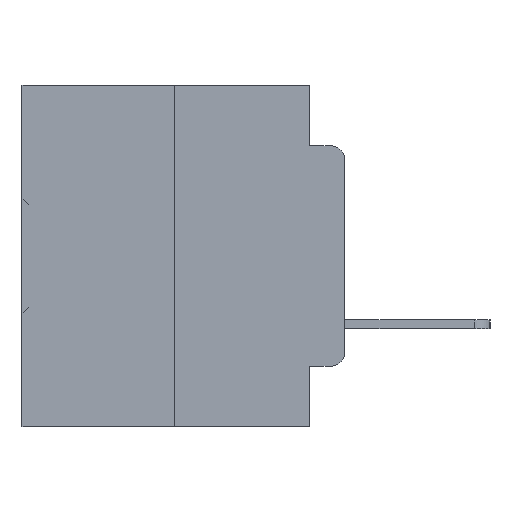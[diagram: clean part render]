
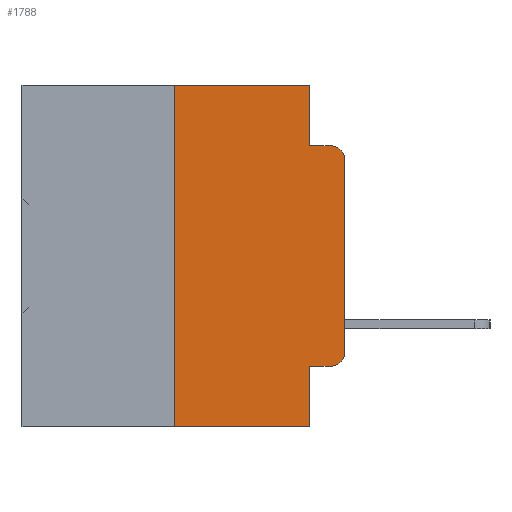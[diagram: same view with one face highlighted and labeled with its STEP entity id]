
A CAD part, left-side view. The second image highlights one B-rep face of the part: STEP entity #1788.
In plain terms, the highlighted planar face has unit normal (-1, 0, 0).
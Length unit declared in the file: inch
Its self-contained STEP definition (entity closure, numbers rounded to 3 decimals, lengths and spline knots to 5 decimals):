
#322 = CARTESIAN_POINT ( 'NONE',  ( 0., 0., -0.3915 ) ) ;
#651 = VECTOR ( 'NONE', #25806, 39.37008 ) ;
#716 = ORIENTED_EDGE ( 'NONE', *, *, #27039, .T. ) ;
#754 = DIRECTION ( 'NONE',  ( 0., -1., 0. ) ) ;
#1628 = CARTESIAN_POINT ( 'NONE',  ( 0., 0.25, 0. ) ) ;
#1788 = ADVANCED_FACE ( 'NONE', ( #13423 ), #5880, .F. ) ;
#2071 = VERTEX_POINT ( 'NONE', #32839 ) ;
#2243 = LINE ( 'NONE', #10859, #23206 ) ;
#2518 = CIRCLE ( 'NONE', #29534, 0.02 ) ;
#3226 = ORIENTED_EDGE ( 'NONE', *, *, #8585, .F. ) ;
#4117 = CARTESIAN_POINT ( 'NONE',  ( 0., 0.051, -0.0885 ) ) ;
#4327 = VERTEX_POINT ( 'NONE', #17687 ) ;
#4739 = DIRECTION ( 'NONE',  ( 0., 0., -1. ) ) ;
#5241 = DIRECTION ( 'NONE',  ( -1., 0., 0. ) ) ;
#5880 = PLANE ( 'NONE',  #23293 ) ;
#6751 = CARTESIAN_POINT ( 'NONE',  ( 0., 0.051, -0.4115 ) ) ;
#6845 = VERTEX_POINT ( 'NONE', #28659 ) ;
#7398 = LINE ( 'NONE', #20238, #21062 ) ;
#7960 = LINE ( 'NONE', #6751, #651 ) ;
#8549 = DIRECTION ( 'NONE',  ( 0., 0., -1. ) ) ;
#8585 = EDGE_CURVE ( 'NONE', #31777, #33695, #7398, .T. ) ;
#8704 = DIRECTION ( 'NONE',  ( 0., 0., -1. ) ) ;
#10718 = DIRECTION ( 'NONE',  ( 0., -1., 0. ) ) ;
#10859 = CARTESIAN_POINT ( 'NONE',  ( 0., 0., 0. ) ) ;
#11334 = DIRECTION ( 'NONE',  ( 1., 0., 0. ) ) ;
#11794 = DIRECTION ( 'NONE',  ( -1., 0., 0. ) ) ;
#12332 = EDGE_CURVE ( 'NONE', #2071, #6845, #7960, .T. ) ;
#12354 = LINE ( 'NONE', #27986, #25967 ) ;
#12371 = DIRECTION ( 'NONE',  ( 0., -1., 0. ) ) ;
#13351 = VERTEX_POINT ( 'NONE', #322 ) ;
#13352 = CARTESIAN_POINT ( 'NONE',  ( 0., 0.051, 0. ) ) ;
#13423 = FACE_OUTER_BOUND ( 'NONE', #16898, .T. ) ;
#13472 = EDGE_CURVE ( 'NONE', #6845, #13351, #27029, .T. ) ;
#13882 = VERTEX_POINT ( 'NONE', #32390 ) ;
#14518 = DIRECTION ( 'NONE',  ( 0., 0., 1. ) ) ;
#14878 = EDGE_CURVE ( 'NONE', #2071, #4327, #18936, .T. ) ;
#15846 = VERTEX_POINT ( 'NONE', #20016 ) ;
#16189 = EDGE_CURVE ( 'NONE', #15846, #13882, #2518, .T. ) ;
#16545 = ORIENTED_EDGE ( 'NONE', *, *, #29329, .F. ) ;
#16795 = CARTESIAN_POINT ( 'NONE',  ( 0., 0.473, 0. ) ) ;
#16898 = EDGE_LOOP ( 'NONE', ( #716, #28447, #17100, #18820, #3226, #16545, #24313, #28804, #24679, #28903 ) ) ;
#17100 = ORIENTED_EDGE ( 'NONE', *, *, #19858, .F. ) ;
#17377 = VECTOR ( 'NONE', #754, 39.37008 ) ;
#17687 = CARTESIAN_POINT ( 'NONE',  ( 0., 0.051, -0.5 ) ) ;
#17875 = EDGE_CURVE ( 'NONE', #33695, #21159, #27769, .T. ) ;
#18107 = VECTOR ( 'NONE', #4739, 39.37008 ) ;
#18820 = ORIENTED_EDGE ( 'NONE', *, *, #17875, .F. ) ;
#18852 = CARTESIAN_POINT ( 'NONE',  ( 0., 0.051, -0.0885 ) ) ;
#18936 = LINE ( 'NONE', #29202, #18107 ) ;
#19195 = VECTOR ( 'NONE', #12371, 39.37008 ) ;
#19858 = EDGE_CURVE ( 'NONE', #21159, #13882, #27189, .T. ) ;
#20016 = CARTESIAN_POINT ( 'NONE',  ( 0., 0., -0.1085 ) ) ;
#20238 = CARTESIAN_POINT ( 'NONE',  ( 0., 0.473, 0. ) ) ;
#21062 = VECTOR ( 'NONE', #10718, 39.37008 ) ;
#21159 = VERTEX_POINT ( 'NONE', #18852 ) ;
#21637 = CARTESIAN_POINT ( 'NONE',  ( 0., 0.02, -0.1085 ) ) ;
#21879 = DIRECTION ( 'NONE',  ( 0., 0., 1. ) ) ;
#23206 = VECTOR ( 'NONE', #21879, 39.37008 ) ;
#23293 = AXIS2_PLACEMENT_3D ( 'NONE', #16795, #11334, #8549 ) ;
#24313 = ORIENTED_EDGE ( 'NONE', *, *, #32146, .T. ) ;
#24346 = DIRECTION ( 'NONE',  ( 0., 0., -1. ) ) ;
#24679 = ORIENTED_EDGE ( 'NONE', *, *, #12332, .T. ) ;
#25471 = CARTESIAN_POINT ( 'NONE',  ( 0., 0.25, -0.5 ) ) ;
#25806 = DIRECTION ( 'NONE',  ( 0., -1., 0. ) ) ;
#25967 = VECTOR ( 'NONE', #14518, 39.37008 ) ;
#26474 = AXIS2_PLACEMENT_3D ( 'NONE', #28043, #11794, #30707 ) ;
#27029 = CIRCLE ( 'NONE', #26474, 0.02 ) ;
#27039 = EDGE_CURVE ( 'NONE', #13351, #15846, #2243, .T. ) ;
#27189 = LINE ( 'NONE', #4117, #19195 ) ;
#27769 = LINE ( 'NONE', #32873, #33934 ) ;
#27834 = VERTEX_POINT ( 'NONE', #25471 ) ;
#27986 = CARTESIAN_POINT ( 'NONE',  ( 0., 0.25, 0. ) ) ;
#28043 = CARTESIAN_POINT ( 'NONE',  ( 0., 0.02, -0.3915 ) ) ;
#28447 = ORIENTED_EDGE ( 'NONE', *, *, #16189, .T. ) ;
#28659 = CARTESIAN_POINT ( 'NONE',  ( 0., 0.02, -0.4115 ) ) ;
#28804 = ORIENTED_EDGE ( 'NONE', *, *, #14878, .F. ) ;
#28903 = ORIENTED_EDGE ( 'NONE', *, *, #13472, .T. ) ;
#29202 = CARTESIAN_POINT ( 'NONE',  ( 0., 0.051, 0. ) ) ;
#29329 = EDGE_CURVE ( 'NONE', #27834, #31777, #12354, .T. ) ;
#29534 = AXIS2_PLACEMENT_3D ( 'NONE', #21637, #5241, #24346 ) ;
#30537 = CARTESIAN_POINT ( 'NONE',  ( 0., 0.473, -0.5 ) ) ;
#30707 = DIRECTION ( 'NONE',  ( 0., 0., -1. ) ) ;
#31627 = LINE ( 'NONE', #30537, #17377 ) ;
#31777 = VERTEX_POINT ( 'NONE', #1628 ) ;
#32146 = EDGE_CURVE ( 'NONE', #27834, #4327, #31627, .T. ) ;
#32390 = CARTESIAN_POINT ( 'NONE',  ( 0., 0.02, -0.0885 ) ) ;
#32839 = CARTESIAN_POINT ( 'NONE',  ( 0., 0.051, -0.4115 ) ) ;
#32873 = CARTESIAN_POINT ( 'NONE',  ( 0., 0.051, 0. ) ) ;
#33695 = VERTEX_POINT ( 'NONE', #13352 ) ;
#33934 = VECTOR ( 'NONE', #8704, 39.37008 ) ;
